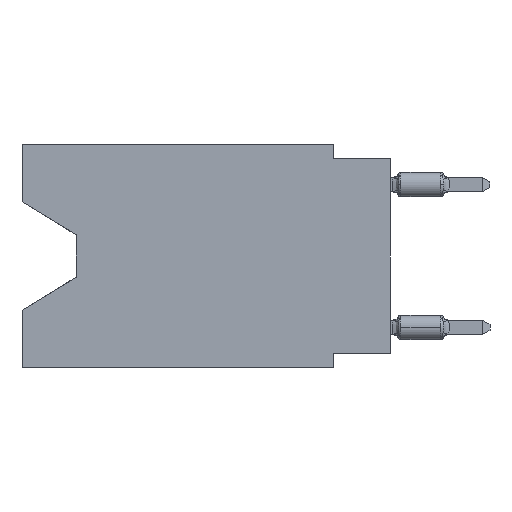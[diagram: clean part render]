
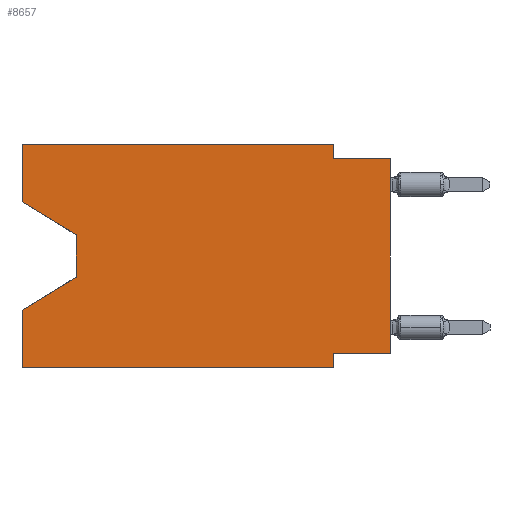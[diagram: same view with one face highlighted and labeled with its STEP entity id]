
A CAD part, left-side view. The second image highlights one B-rep face of the part: STEP entity #8657.
In plain terms, the highlighted planar face has unit normal (-1, 0, 0).
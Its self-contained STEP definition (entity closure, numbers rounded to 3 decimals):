
#206 = DIRECTION ( 'NONE',  ( 0., -1., 0. ) ) ;
#303 = LINE ( 'NONE', #7255, #15265 ) ;
#593 = VERTEX_POINT ( 'NONE', #3201 ) ;
#700 = VECTOR ( 'NONE', #1802, 1000. ) ;
#762 = VERTEX_POINT ( 'NONE', #9569 ) ;
#1212 = ORIENTED_EDGE ( 'NONE', *, *, #4526, .T. ) ;
#1253 = CARTESIAN_POINT ( 'NONE',  ( 0., 2.54, 0. ) ) ;
#1256 = CARTESIAN_POINT ( 'NONE',  ( 0., 16.383, 0. ) ) ;
#1279 = VERTEX_POINT ( 'NONE', #5334 ) ;
#1754 = VERTEX_POINT ( 'NONE', #1253 ) ;
#1772 = ORIENTED_EDGE ( 'NONE', *, *, #15750, .T. ) ;
#1802 = DIRECTION ( 'NONE',  ( 0., 0., -1. ) ) ;
#1903 = CARTESIAN_POINT ( 'NONE',  ( 0., 16.383, -9.906 ) ) ;
#1930 = CARTESIAN_POINT ( 'NONE',  ( 0., 2.54, -0.635 ) ) ;
#2068 = DIRECTION ( 'NONE',  ( 0., -0.855, -0.519 ) ) ;
#2252 = ORIENTED_EDGE ( 'NONE', *, *, #3412, .T. ) ;
#2650 = LINE ( 'NONE', #12439, #4378 ) ;
#2881 = VERTEX_POINT ( 'NONE', #15201 ) ;
#3185 = LINE ( 'NONE', #7311, #6736 ) ;
#3201 = CARTESIAN_POINT ( 'NONE',  ( 0., 2.54, -9.906 ) ) ;
#3412 = EDGE_CURVE ( 'NONE', #15962, #762, #2650, .T. ) ;
#3504 = LINE ( 'NONE', #1903, #17527 ) ;
#3804 = LINE ( 'NONE', #7662, #4011 ) ;
#3885 = EDGE_CURVE ( 'NONE', #14941, #762, #16099, .T. ) ;
#3997 = CARTESIAN_POINT ( 'NONE',  ( 0., 16.383, 0. ) ) ;
#4011 = VECTOR ( 'NONE', #7842, 1000. ) ;
#4042 = VECTOR ( 'NONE', #2068, 1000. ) ;
#4192 = CARTESIAN_POINT ( 'NONE',  ( 0., 0., -9.271 ) ) ;
#4378 = VECTOR ( 'NONE', #8300, 1000. ) ;
#4437 = EDGE_LOOP ( 'NONE', ( #1212, #1772, #5051, #8784, #17570, #15707, #17624, #2252, #11360, #14673, #16265, #8419 ) ) ;
#4526 = EDGE_CURVE ( 'NONE', #6223, #1279, #10980, .T. ) ;
#5051 = ORIENTED_EDGE ( 'NONE', *, *, #8031, .T. ) ;
#5334 = CARTESIAN_POINT ( 'NONE',  ( 0., 13.97, -4.013 ) ) ;
#5855 = DIRECTION ( 'NONE',  ( 0., 1., 0. ) ) ;
#5935 = EDGE_CURVE ( 'NONE', #15996, #1754, #17087, .T. ) ;
#6223 = VERTEX_POINT ( 'NONE', #6730 ) ;
#6432 = EDGE_CURVE ( 'NONE', #1754, #14941, #3804, .T. ) ;
#6643 = EDGE_CURVE ( 'NONE', #2881, #593, #12909, .T. ) ;
#6730 = CARTESIAN_POINT ( 'NONE',  ( 0., 16.383, -2.546 ) ) ;
#6736 = VECTOR ( 'NONE', #7598, 1000. ) ;
#7211 = CARTESIAN_POINT ( 'NONE',  ( 0., 16.383, 0. ) ) ;
#7255 = CARTESIAN_POINT ( 'NONE',  ( 0., 0., -9.271 ) ) ;
#7311 = CARTESIAN_POINT ( 'NONE',  ( 0., 13.97, -5.893 ) ) ;
#7526 = DIRECTION ( 'NONE',  ( 0., -1., 0. ) ) ;
#7598 = DIRECTION ( 'NONE',  ( 0., 0.855, -0.519 ) ) ;
#7662 = CARTESIAN_POINT ( 'NONE',  ( 0., 2.54, 0. ) ) ;
#7724 = CARTESIAN_POINT ( 'NONE',  ( 0., 0., -0.635 ) ) ;
#7754 = CARTESIAN_POINT ( 'NONE',  ( 0., 16.383, -7.36 ) ) ;
#7841 = VECTOR ( 'NONE', #17141, 1000. ) ;
#7842 = DIRECTION ( 'NONE',  ( 0., 0., -1. ) ) ;
#8031 = EDGE_CURVE ( 'NONE', #13231, #11280, #3185, .T. ) ;
#8300 = DIRECTION ( 'NONE',  ( 0., 0., 1. ) ) ;
#8319 = FACE_OUTER_BOUND ( 'NONE', #4437, .T. ) ;
#8408 = LINE ( 'NONE', #1256, #7841 ) ;
#8419 = ORIENTED_EDGE ( 'NONE', *, *, #14311, .F. ) ;
#8632 = LINE ( 'NONE', #12962, #14400 ) ;
#8657 = ADVANCED_FACE ( 'NONE', ( #8319 ), #12651, .F. ) ;
#8784 = ORIENTED_EDGE ( 'NONE', *, *, #13320, .F. ) ;
#9291 = CARTESIAN_POINT ( 'NONE',  ( 0., 16.383, -2.546 ) ) ;
#9569 = CARTESIAN_POINT ( 'NONE',  ( 0., 0., -0.635 ) ) ;
#9939 = DIRECTION ( 'NONE',  ( 0., -1., 0. ) ) ;
#10980 = LINE ( 'NONE', #9291, #4042 ) ;
#11034 = DIRECTION ( 'NONE',  ( 0., 0., -1. ) ) ;
#11280 = VERTEX_POINT ( 'NONE', #7754 ) ;
#11360 = ORIENTED_EDGE ( 'NONE', *, *, #3885, .F. ) ;
#11583 = CARTESIAN_POINT ( 'NONE',  ( 0., 2.54, -9.906 ) ) ;
#11632 = DIRECTION ( 'NONE',  ( 0., 0., -1. ) ) ;
#11672 = EDGE_CURVE ( 'NONE', #14194, #593, #3504, .T. ) ;
#11753 = LINE ( 'NONE', #16093, #12319 ) ;
#11800 = CARTESIAN_POINT ( 'NONE',  ( 0., 16.383, 0. ) ) ;
#12195 = CARTESIAN_POINT ( 'NONE',  ( 0., 16.383, -9.906 ) ) ;
#12319 = VECTOR ( 'NONE', #16554, 1000. ) ;
#12439 = CARTESIAN_POINT ( 'NONE',  ( 0., 0., 0. ) ) ;
#12651 = PLANE ( 'NONE',  #17253 ) ;
#12909 = LINE ( 'NONE', #11583, #700 ) ;
#12962 = CARTESIAN_POINT ( 'NONE',  ( 0., 13.97, -4.013 ) ) ;
#13231 = VERTEX_POINT ( 'NONE', #15991 ) ;
#13295 = VECTOR ( 'NONE', #9939, 1000. ) ;
#13320 = EDGE_CURVE ( 'NONE', #14194, #11280, #11753, .T. ) ;
#14150 = DIRECTION ( 'NONE',  ( 1., 0., 0. ) ) ;
#14194 = VERTEX_POINT ( 'NONE', #12195 ) ;
#14311 = EDGE_CURVE ( 'NONE', #6223, #15996, #8408, .T. ) ;
#14400 = VECTOR ( 'NONE', #11632, 1000. ) ;
#14673 = ORIENTED_EDGE ( 'NONE', *, *, #6432, .F. ) ;
#14842 = VECTOR ( 'NONE', #7526, 1000. ) ;
#14941 = VERTEX_POINT ( 'NONE', #1930 ) ;
#15201 = CARTESIAN_POINT ( 'NONE',  ( 0., 2.54, -9.271 ) ) ;
#15265 = VECTOR ( 'NONE', #5855, 1000. ) ;
#15707 = ORIENTED_EDGE ( 'NONE', *, *, #6643, .F. ) ;
#15750 = EDGE_CURVE ( 'NONE', #1279, #13231, #8632, .T. ) ;
#15962 = VERTEX_POINT ( 'NONE', #4192 ) ;
#15991 = CARTESIAN_POINT ( 'NONE',  ( 0., 13.97, -5.893 ) ) ;
#15996 = VERTEX_POINT ( 'NONE', #11800 ) ;
#16093 = CARTESIAN_POINT ( 'NONE',  ( 0., 16.383, 0. ) ) ;
#16099 = LINE ( 'NONE', #7724, #14842 ) ;
#16265 = ORIENTED_EDGE ( 'NONE', *, *, #5935, .F. ) ;
#16554 = DIRECTION ( 'NONE',  ( 0., 0., 1. ) ) ;
#17087 = LINE ( 'NONE', #7211, #13295 ) ;
#17141 = DIRECTION ( 'NONE',  ( 0., 0., 1. ) ) ;
#17253 = AXIS2_PLACEMENT_3D ( 'NONE', #3997, #14150, #11034 ) ;
#17527 = VECTOR ( 'NONE', #206, 1000. ) ;
#17570 = ORIENTED_EDGE ( 'NONE', *, *, #11672, .T. ) ;
#17624 = ORIENTED_EDGE ( 'NONE', *, *, #17685, .F. ) ;
#17685 = EDGE_CURVE ( 'NONE', #15962, #2881, #303, .T. ) ;
